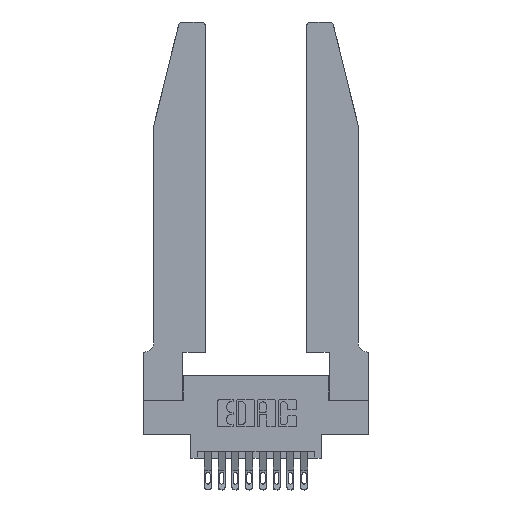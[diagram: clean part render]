
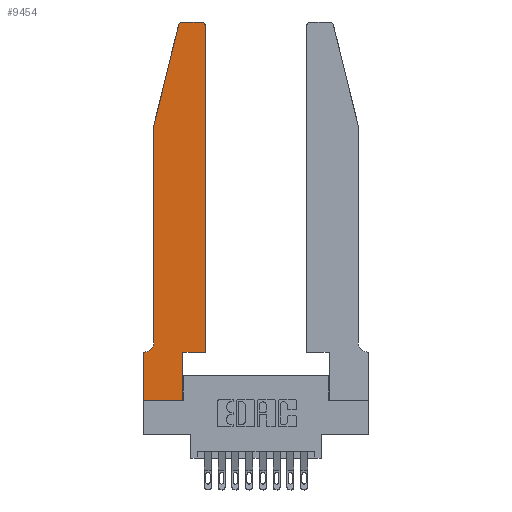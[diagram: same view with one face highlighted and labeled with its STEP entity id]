
A CAD part, top view. The second image highlights one B-rep face of the part: STEP entity #9454.
In plain terms, the highlighted planar face has unit normal (0, 0, 1).
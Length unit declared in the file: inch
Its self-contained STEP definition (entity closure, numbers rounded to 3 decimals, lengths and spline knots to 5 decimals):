
#69 = DIRECTION ( 'NONE',  ( 1., 0., 0. ) ) ;
#84 = CARTESIAN_POINT ( 'NONE',  ( 0.2865, 0.35, 0.37 ) ) ;
#133 = CARTESIAN_POINT ( 'NONE',  ( 0.25487, 2.72718, 0.37 ) ) ;
#193 = LINE ( 'NONE', #11979, #13463 ) ;
#249 = EDGE_CURVE ( 'NONE', #14077, #11343, #12452, .T. ) ;
#665 = CARTESIAN_POINT ( 'NONE',  ( 0.0055, 0.35, 0.37 ) ) ;
#671 = EDGE_CURVE ( 'NONE', #9458, #11762, #7805, .T. ) ;
#1270 = ORIENTED_EDGE ( 'NONE', *, *, #3301, .T. ) ;
#1280 = DIRECTION ( 'NONE',  ( 0., 0., 1. ) ) ;
#1726 = CARTESIAN_POINT ( 'NONE',  ( 0.4205, 2.72, 0.37 ) ) ;
#2125 = CARTESIAN_POINT ( 'NONE',  ( 0.2865, 0., 0.37 ) ) ;
#2434 = DIRECTION ( 'NONE',  ( -0.239, -0.971, 0. ) ) ;
#2491 = DIRECTION ( 'NONE',  ( -1., 0., 0. ) ) ;
#2850 = CARTESIAN_POINT ( 'NONE',  ( 0.2865, 0.35, 0.37 ) ) ;
#2887 = EDGE_CURVE ( 'NONE', #5539, #11608, #7548, .T. ) ;
#2979 = LINE ( 'NONE', #3830, #6709 ) ;
#3164 = FACE_OUTER_BOUND ( 'NONE', #15282, .T. ) ;
#3298 = VECTOR ( 'NONE', #15844, 39.37008 ) ;
#3301 = EDGE_CURVE ( 'NONE', #5524, #5539, #10768, .T. ) ;
#3481 = DIRECTION ( 'NONE',  ( 0., 0., 1. ) ) ;
#3530 = VERTEX_POINT ( 'NONE', #14920 ) ;
#3696 = LINE ( 'NONE', #8529, #3298 ) ;
#3802 = CARTESIAN_POINT ( 'NONE',  ( 0.0755, 0.35, 0.37 ) ) ;
#3805 = LINE ( 'NONE', #14346, #10845 ) ;
#3830 = CARTESIAN_POINT ( 'NONE',  ( 0., 0., 0.37 ) ) ;
#3928 = CARTESIAN_POINT ( 'NONE',  ( 0., 0., 0.37 ) ) ;
#3937 = DIRECTION ( 'NONE',  ( 1., 0., 0. ) ) ;
#3947 = VERTEX_POINT ( 'NONE', #15929 ) ;
#4155 = ORIENTED_EDGE ( 'NONE', *, *, #6912, .T. ) ;
#4392 = ORIENTED_EDGE ( 'NONE', *, *, #671, .T. ) ;
#4494 = DIRECTION ( 'NONE',  ( 0., 1., 0. ) ) ;
#4829 = ORIENTED_EDGE ( 'NONE', *, *, #13189, .T. ) ;
#5524 = VERTEX_POINT ( 'NONE', #11383 ) ;
#5539 = VERTEX_POINT ( 'NONE', #133 ) ;
#6074 = CARTESIAN_POINT ( 'NONE',  ( 0.0055, 0.42, 0.37 ) ) ;
#6709 = VECTOR ( 'NONE', #69, 39.37008 ) ;
#6912 = EDGE_CURVE ( 'NONE', #9545, #7886, #3805, .T. ) ;
#6995 = DIRECTION ( 'NONE',  ( 0., -1., 0. ) ) ;
#7372 = DIRECTION ( 'NONE',  ( -1., 0., 0. ) ) ;
#7548 = LINE ( 'NONE', #9915, #10846 ) ;
#7783 = AXIS2_PLACEMENT_3D ( 'NONE', #6074, #14695, #7372 ) ;
#7805 = LINE ( 'NONE', #84, #14328 ) ;
#7886 = VERTEX_POINT ( 'NONE', #3928 ) ;
#8350 = DIRECTION ( 'NONE',  ( 1., 0., 0. ) ) ;
#8362 = EDGE_CURVE ( 'NONE', #11343, #5524, #11197, .T. ) ;
#8456 = EDGE_CURVE ( 'NONE', #7886, #9458, #2979, .T. ) ;
#8529 = CARTESIAN_POINT ( 'NONE',  ( 0.4505, 0.35, 0.37 ) ) ;
#8550 = AXIS2_PLACEMENT_3D ( 'NONE', #12025, #15671, #8350 ) ;
#8723 = CARTESIAN_POINT ( 'NONE',  ( 0.2605, 2.75, 0.37 ) ) ;
#8768 = CARTESIAN_POINT ( 'NONE',  ( 0.0755, 2., 0.37 ) ) ;
#9176 = ORIENTED_EDGE ( 'NONE', *, *, #249, .T. ) ;
#9438 = ORIENTED_EDGE ( 'NONE', *, *, #10838, .T. ) ;
#9454 = ADVANCED_FACE ( 'NONE', ( #3164 ), #14407, .T. ) ;
#9458 = VERTEX_POINT ( 'NONE', #2125 ) ;
#9545 = VERTEX_POINT ( 'NONE', #9833 ) ;
#9643 = DIRECTION ( 'NONE',  ( 0., 1., 0. ) ) ;
#9833 = CARTESIAN_POINT ( 'NONE',  ( 0., 0.35, 0.37 ) ) ;
#9915 = CARTESIAN_POINT ( 'NONE',  ( 0.0755, 2., 0.37 ) ) ;
#9919 = VECTOR ( 'NONE', #13551, 39.37008 ) ;
#10044 = VECTOR ( 'NONE', #2491, 39.37008 ) ;
#10299 = ORIENTED_EDGE ( 'NONE', *, *, #13701, .T. ) ;
#10768 = CIRCLE ( 'NONE', #15965, 0.03 ) ;
#10838 = EDGE_CURVE ( 'NONE', #3530, #14077, #193, .T. ) ;
#10845 = VECTOR ( 'NONE', #6995, 39.37008 ) ;
#10846 = VECTOR ( 'NONE', #2434, 39.37008 ) ;
#10961 = CARTESIAN_POINT ( 'NONE',  ( 0.284, 2.72, 0.37 ) ) ;
#11149 = CIRCLE ( 'NONE', #7783, 0.07 ) ;
#11197 = LINE ( 'NONE', #8723, #10044 ) ;
#11342 = ORIENTED_EDGE ( 'NONE', *, *, #15650, .T. ) ;
#11343 = VERTEX_POINT ( 'NONE', #14391 ) ;
#11383 = CARTESIAN_POINT ( 'NONE',  ( 0.284, 2.75, 0.37 ) ) ;
#11544 = ORIENTED_EDGE ( 'NONE', *, *, #2887, .T. ) ;
#11608 = VERTEX_POINT ( 'NONE', #8768 ) ;
#11717 = CARTESIAN_POINT ( 'NONE',  ( 0.4505, 2.72, 0.37 ) ) ;
#11762 = VERTEX_POINT ( 'NONE', #2850 ) ;
#11979 = CARTESIAN_POINT ( 'NONE',  ( 0.4505, 0.35, 0.37 ) ) ;
#12025 = CARTESIAN_POINT ( 'NONE',  ( 0., 0.35, 0.37 ) ) ;
#12186 = DIRECTION ( 'NONE',  ( 1., 0., 0. ) ) ;
#12260 = DIRECTION ( 'NONE',  ( -1., 0., 0. ) ) ;
#12273 = ORIENTED_EDGE ( 'NONE', *, *, #8456, .T. ) ;
#12449 = ORIENTED_EDGE ( 'NONE', *, *, #8362, .T. ) ;
#12452 = CIRCLE ( 'NONE', #14541, 0.03 ) ;
#12713 = ORIENTED_EDGE ( 'NONE', *, *, #15741, .T. ) ;
#12763 = LINE ( 'NONE', #3802, #15228 ) ;
#13145 = LINE ( 'NONE', #14715, #9919 ) ;
#13189 = EDGE_CURVE ( 'NONE', #3947, #16078, #11149, .T. ) ;
#13463 = VECTOR ( 'NONE', #4494, 39.37008 ) ;
#13551 = DIRECTION ( 'NONE',  ( 0., -1., 0. ) ) ;
#13701 = EDGE_CURVE ( 'NONE', #11762, #3530, #3696, .T. ) ;
#14077 = VERTEX_POINT ( 'NONE', #11717 ) ;
#14328 = VECTOR ( 'NONE', #9643, 39.37008 ) ;
#14346 = CARTESIAN_POINT ( 'NONE',  ( 0., 0., 0.37 ) ) ;
#14391 = CARTESIAN_POINT ( 'NONE',  ( 0.4205, 2.75, 0.37 ) ) ;
#14407 = PLANE ( 'NONE',  #8550 ) ;
#14541 = AXIS2_PLACEMENT_3D ( 'NONE', #1726, #1280, #3937 ) ;
#14695 = DIRECTION ( 'NONE',  ( 0., 0., -1. ) ) ;
#14715 = CARTESIAN_POINT ( 'NONE',  ( 0.0755, 2., 0.37 ) ) ;
#14920 = CARTESIAN_POINT ( 'NONE',  ( 0.4505, 0.35, 0.37 ) ) ;
#15228 = VECTOR ( 'NONE', #12260, 39.37008 ) ;
#15282 = EDGE_LOOP ( 'NONE', ( #12449, #1270, #11544, #11342, #4829, #12713, #4155, #12273, #4392, #10299, #9438, #9176 ) ) ;
#15650 = EDGE_CURVE ( 'NONE', #11608, #3947, #13145, .T. ) ;
#15671 = DIRECTION ( 'NONE',  ( 0., 0., 1. ) ) ;
#15741 = EDGE_CURVE ( 'NONE', #16078, #9545, #12763, .T. ) ;
#15844 = DIRECTION ( 'NONE',  ( 1., 0., 0. ) ) ;
#15929 = CARTESIAN_POINT ( 'NONE',  ( 0.0755, 0.42, 0.37 ) ) ;
#15965 = AXIS2_PLACEMENT_3D ( 'NONE', #10961, #3481, #12186 ) ;
#16078 = VERTEX_POINT ( 'NONE', #665 ) ;
